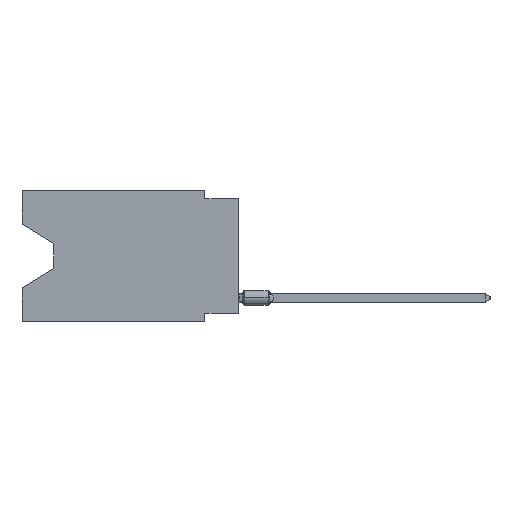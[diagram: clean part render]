
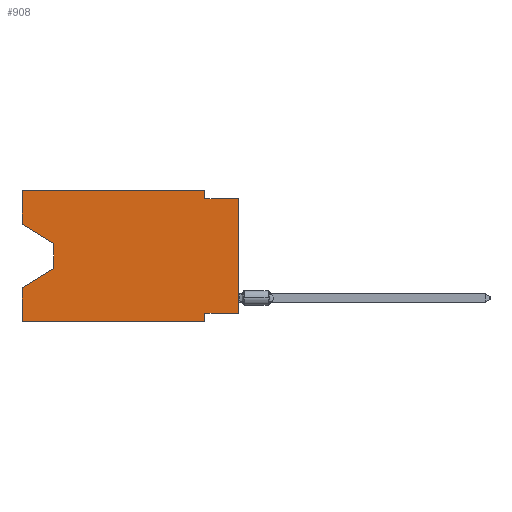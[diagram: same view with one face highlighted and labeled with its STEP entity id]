
A CAD part, left-side view. The second image highlights one B-rep face of the part: STEP entity #908.
In plain terms, the highlighted planar face has unit normal (-1, 0, 0).
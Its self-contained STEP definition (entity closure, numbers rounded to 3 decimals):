
#714 = VECTOR ( 'NONE', #26405, 1000. ) ;
#908 = ADVANCED_FACE ( 'NONE', ( #21425 ), #6537, .F. ) ;
#1660 = ORIENTED_EDGE ( 'NONE', *, *, #21030, .F. ) ;
#1944 = LINE ( 'NONE', #29620, #20641 ) ;
#1955 = EDGE_CURVE ( 'NONE', #30553, #7448, #3778, .T. ) ;
#2251 = LINE ( 'NONE', #2651, #38185 ) ;
#2651 = CARTESIAN_POINT ( 'NONE',  ( 0., 16.383, 0. ) ) ;
#2909 = ORIENTED_EDGE ( 'NONE', *, *, #29033, .T. ) ;
#3778 = LINE ( 'NONE', #25559, #18617 ) ;
#4230 = EDGE_CURVE ( 'NONE', #8993, #28546, #26884, .T. ) ;
#4737 = CARTESIAN_POINT ( 'NONE',  ( 0., 2.54, -9.906 ) ) ;
#5143 = CARTESIAN_POINT ( 'NONE',  ( 0., 2.54, -9.906 ) ) ;
#6537 = PLANE ( 'NONE',  #19054 ) ;
#6947 = CARTESIAN_POINT ( 'NONE',  ( 0., 0., 0. ) ) ;
#7448 = VERTEX_POINT ( 'NONE', #33869 ) ;
#7496 = ORIENTED_EDGE ( 'NONE', *, *, #20073, .F. ) ;
#7651 = ORIENTED_EDGE ( 'NONE', *, *, #30023, .F. ) ;
#8011 = CARTESIAN_POINT ( 'NONE',  ( 0., 13.97, -4.013 ) ) ;
#8577 = VECTOR ( 'NONE', #33375, 1000. ) ;
#8962 = CARTESIAN_POINT ( 'NONE',  ( 0., 16.383, 0. ) ) ;
#8993 = VERTEX_POINT ( 'NONE', #18627 ) ;
#9781 = DIRECTION ( 'NONE',  ( 0., 0., -1. ) ) ;
#9821 = VERTEX_POINT ( 'NONE', #38254 ) ;
#10120 = ORIENTED_EDGE ( 'NONE', *, *, #4230, .F. ) ;
#10438 = CARTESIAN_POINT ( 'NONE',  ( 0., 16.383, 0. ) ) ;
#11274 = VECTOR ( 'NONE', #13579, 1000. ) ;
#11291 = VERTEX_POINT ( 'NONE', #8011 ) ;
#11732 = ORIENTED_EDGE ( 'NONE', *, *, #23243, .T. ) ;
#13429 = LINE ( 'NONE', #25865, #39146 ) ;
#13579 = DIRECTION ( 'NONE',  ( 0., 0., -1. ) ) ;
#13972 = LINE ( 'NONE', #29235, #714 ) ;
#14395 = LINE ( 'NONE', #26620, #11274 ) ;
#14803 = VERTEX_POINT ( 'NONE', #4737 ) ;
#15145 = LINE ( 'NONE', #39327, #24315 ) ;
#15314 = CARTESIAN_POINT ( 'NONE',  ( 0., 0., -0.635 ) ) ;
#15354 = EDGE_LOOP ( 'NONE', ( #2909, #30994, #11732, #10120, #25870, #31194, #7496, #32882, #1660, #35806, #24897, #7651 ) ) ;
#15690 = VECTOR ( 'NONE', #20815, 1000. ) ;
#16658 = CARTESIAN_POINT ( 'NONE',  ( 0., 2.54, -9.271 ) ) ;
#17304 = VERTEX_POINT ( 'NONE', #31426 ) ;
#17793 = VERTEX_POINT ( 'NONE', #15314 ) ;
#18617 = VECTOR ( 'NONE', #25159, 1000. ) ;
#18627 = CARTESIAN_POINT ( 'NONE',  ( 0., 16.383, -9.906 ) ) ;
#19054 = AXIS2_PLACEMENT_3D ( 'NONE', #25067, #21831, #9781 ) ;
#19885 = CARTESIAN_POINT ( 'NONE',  ( 0., 16.383, -9.906 ) ) ;
#20073 = EDGE_CURVE ( 'NONE', #17304, #27988, #13429, .T. ) ;
#20600 = EDGE_CURVE ( 'NONE', #11291, #21993, #14395, .T. ) ;
#20641 = VECTOR ( 'NONE', #27180, 1000. ) ;
#20815 = DIRECTION ( 'NONE',  ( 0., 0.855, -0.519 ) ) ;
#21030 = EDGE_CURVE ( 'NONE', #23866, #17793, #15145, .T. ) ;
#21425 = FACE_OUTER_BOUND ( 'NONE', #15354, .T. ) ;
#21494 = EDGE_CURVE ( 'NONE', #27988, #14803, #35822, .T. ) ;
#21801 = CARTESIAN_POINT ( 'NONE',  ( 0., 16.383, -7.36 ) ) ;
#21831 = DIRECTION ( 'NONE',  ( 1., 0., 0. ) ) ;
#21993 = VERTEX_POINT ( 'NONE', #24624 ) ;
#22017 = VECTOR ( 'NONE', #25671, 1000. ) ;
#23243 = EDGE_CURVE ( 'NONE', #21993, #28546, #37687, .T. ) ;
#23866 = VERTEX_POINT ( 'NONE', #28408 ) ;
#24315 = VECTOR ( 'NONE', #24530, 1000. ) ;
#24530 = DIRECTION ( 'NONE',  ( 0., -1., 0. ) ) ;
#24624 = CARTESIAN_POINT ( 'NONE',  ( 0., 13.97, -5.893 ) ) ;
#24897 = ORIENTED_EDGE ( 'NONE', *, *, #1955, .F. ) ;
#25067 = CARTESIAN_POINT ( 'NONE',  ( 0., 16.383, 0. ) ) ;
#25159 = DIRECTION ( 'NONE',  ( 0., -1., 0. ) ) ;
#25309 = EDGE_CURVE ( 'NONE', #8993, #14803, #26600, .T. ) ;
#25559 = CARTESIAN_POINT ( 'NONE',  ( 0., 16.383, 0. ) ) ;
#25671 = DIRECTION ( 'NONE',  ( 0., 0., 1. ) ) ;
#25865 = CARTESIAN_POINT ( 'NONE',  ( 0., 0., -9.271 ) ) ;
#25870 = ORIENTED_EDGE ( 'NONE', *, *, #25309, .T. ) ;
#26405 = DIRECTION ( 'NONE',  ( 0., 0., -1. ) ) ;
#26600 = LINE ( 'NONE', #19885, #37843 ) ;
#26620 = CARTESIAN_POINT ( 'NONE',  ( 0., 13.97, -4.013 ) ) ;
#26884 = LINE ( 'NONE', #8962, #8577 ) ;
#27180 = DIRECTION ( 'NONE',  ( 0., -0.855, -0.519 ) ) ;
#27988 = VERTEX_POINT ( 'NONE', #16658 ) ;
#28320 = LINE ( 'NONE', #6947, #22017 ) ;
#28408 = CARTESIAN_POINT ( 'NONE',  ( 0., 2.54, -0.635 ) ) ;
#28546 = VERTEX_POINT ( 'NONE', #21801 ) ;
#29033 = EDGE_CURVE ( 'NONE', #9821, #11291, #1944, .T. ) ;
#29230 = DIRECTION ( 'NONE',  ( 0., -1., 0. ) ) ;
#29235 = CARTESIAN_POINT ( 'NONE',  ( 0., 2.54, 0. ) ) ;
#29620 = CARTESIAN_POINT ( 'NONE',  ( 0., 16.383, -2.546 ) ) ;
#29669 = EDGE_CURVE ( 'NONE', #17304, #17793, #28320, .T. ) ;
#30023 = EDGE_CURVE ( 'NONE', #9821, #30553, #2251, .T. ) ;
#30553 = VERTEX_POINT ( 'NONE', #10438 ) ;
#30994 = ORIENTED_EDGE ( 'NONE', *, *, #20600, .T. ) ;
#31194 = ORIENTED_EDGE ( 'NONE', *, *, #21494, .F. ) ;
#31426 = CARTESIAN_POINT ( 'NONE',  ( 0., 0., -9.271 ) ) ;
#32882 = ORIENTED_EDGE ( 'NONE', *, *, #29669, .T. ) ;
#33194 = DIRECTION ( 'NONE',  ( 0., 0., -1. ) ) ;
#33375 = DIRECTION ( 'NONE',  ( 0., 0., 1. ) ) ;
#33869 = CARTESIAN_POINT ( 'NONE',  ( 0., 2.54, 0. ) ) ;
#34640 = CARTESIAN_POINT ( 'NONE',  ( 0., 13.97, -5.893 ) ) ;
#34921 = EDGE_CURVE ( 'NONE', #7448, #23866, #13972, .T. ) ;
#35806 = ORIENTED_EDGE ( 'NONE', *, *, #34921, .F. ) ;
#35822 = LINE ( 'NONE', #5143, #37313 ) ;
#37004 = DIRECTION ( 'NONE',  ( 0., 0., 1. ) ) ;
#37313 = VECTOR ( 'NONE', #33194, 1000. ) ;
#37687 = LINE ( 'NONE', #34640, #15690 ) ;
#37843 = VECTOR ( 'NONE', #29230, 1000. ) ;
#38185 = VECTOR ( 'NONE', #37004, 1000. ) ;
#38228 = DIRECTION ( 'NONE',  ( 0., 1., 0. ) ) ;
#38254 = CARTESIAN_POINT ( 'NONE',  ( 0., 16.383, -2.546 ) ) ;
#39146 = VECTOR ( 'NONE', #38228, 1000. ) ;
#39327 = CARTESIAN_POINT ( 'NONE',  ( 0., 0., -0.635 ) ) ;
